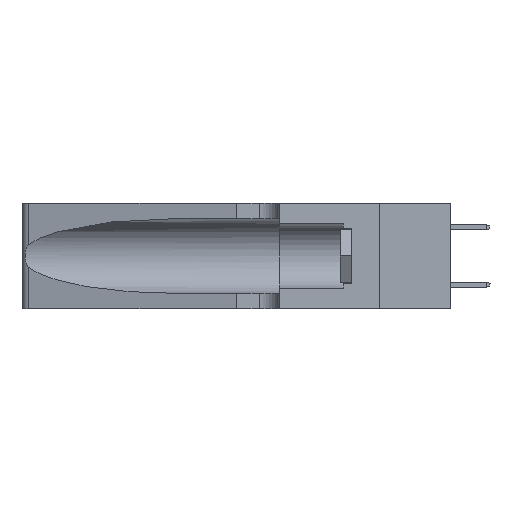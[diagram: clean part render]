
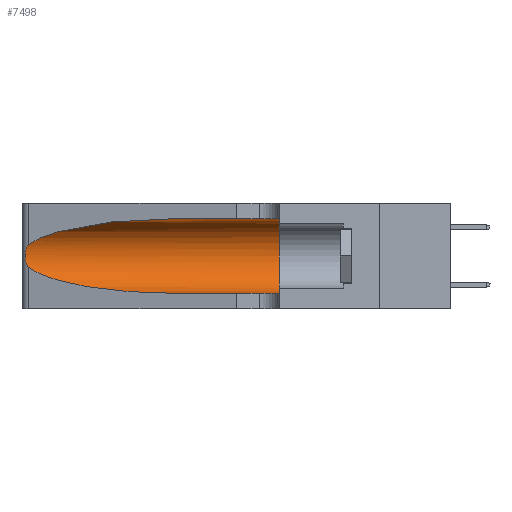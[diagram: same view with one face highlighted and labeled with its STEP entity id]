
A CAD part, left-side view. The second image highlights one B-rep face of the part: STEP entity #7498.
In plain terms, the highlighted cylindrical face has radius 3.308 mm (diameter 6.617 mm), a partial arc.
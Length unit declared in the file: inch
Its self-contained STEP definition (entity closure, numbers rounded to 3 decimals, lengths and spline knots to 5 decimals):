
#547 = VERTEX_POINT ( 'NONE', #1142 ) ;
#1142 = CARTESIAN_POINT ( 'NONE',  ( 0.1305, 0.35, 0.31525 ) ) ;
#2808 = EDGE_LOOP ( 'NONE', ( #38016, #16849, #42690, #29971, #17967, #29332 ) ) ;
#3429 = CARTESIAN_POINT ( 'NONE',  ( 0.25789, 1.23486, 0.15765 ) ) ;
#3972 = CARTESIAN_POINT ( 'NONE',  ( 0.1305, 0.35, 0.05475 ) ) ;
#4000 = FACE_OUTER_BOUND ( 'NONE', #2808, .T. ) ;
#4314 = LINE ( 'NONE', #31258, #21707 ) ;
#4400 = VERTEX_POINT ( 'NONE', #43314 ) ;
#4845 = VERTEX_POINT ( 'NONE', #33265 ) ;
#5397 = CARTESIAN_POINT ( 'NONE',  ( 0.25487, 1.22718, 0.14631 ) ) ;
#5661 = DIRECTION ( 'NONE',  ( 0., 0., 1. ) ) ;
#5883 = CARTESIAN_POINT ( 'NONE',  ( 0.1305, 0.35, 0.185 ) ) ;
#6514 = CARTESIAN_POINT ( 'NONE',  ( 0.25487, 1.22718, 0.22369 ) ) ;
#7188 = CARTESIAN_POINT ( 'NONE',  ( 0.26075, 1.23896, 0.19203 ) ) ;
#7498 = ADVANCED_FACE ( 'NONE', ( #4000 ), #20192, .F. ) ;
#9838 = CARTESIAN_POINT ( 'NONE',  ( 0.18966, 0.96281, 0.31525 ) ) ;
#10511 = CARTESIAN_POINT ( 'NONE',  ( 0.26075, 1.23896, 0.178 ) ) ;
#10900 =( BOUNDED_CURVE ( )  B_SPLINE_CURVE ( 3, ( #19820, #9838, #40145, #18957 ),
 .UNSPECIFIED., .F., .T. ) 
 B_SPLINE_CURVE_WITH_KNOTS ( ( 4, 4 ),
 ( 1.5708, 2.84003 ),
 .UNSPECIFIED. ) 
 CURVE ( )  GEOMETRIC_REPRESENTATION_ITEM ( )  RATIONAL_B_SPLINE_CURVE ( ( 1., 0.87, 0.87, 1. ) ) 
 REPRESENTATION_ITEM ( '' )  );
#13838 = CARTESIAN_POINT ( 'NONE',  ( 0.25639, 1.23184, 0.21858 ) ) ;
#14040 = CARTESIAN_POINT ( 'NONE',  ( 0.26018, 1.23835, 0.19895 ) ) ;
#14261 = CARTESIAN_POINT ( 'NONE',  ( 0.25854, 1.2359, 0.20912 ) ) ;
#16284 = LINE ( 'NONE', #29519, #17554 ) ;
#16849 = ORIENTED_EDGE ( 'NONE', *, *, #32313, .T. ) ;
#16871 = DIRECTION ( 'NONE',  ( 0., 0., -1. ) ) ;
#16875 = CARTESIAN_POINT ( 'NONE',  ( 0.25487, 1.22718, 0.14631 ) ) ;
#17175 = CARTESIAN_POINT ( 'NONE',  ( 0.25555, 1.22994, 0.2215 ) ) ;
#17521 = CARTESIAN_POINT ( 'NONE',  ( 0.1305, 1.61858, 0.185 ) ) ;
#17554 = VECTOR ( 'NONE', #43019, 39.37008 ) ;
#17967 = ORIENTED_EDGE ( 'NONE', *, *, #40953, .F. ) ;
#18218 = VERTEX_POINT ( 'NONE', #16875 ) ;
#18957 = CARTESIAN_POINT ( 'NONE',  ( 0.25487, 1.22718, 0.22369 ) ) ;
#19820 = CARTESIAN_POINT ( 'NONE',  ( 0.1305, 0.72297, 0.31525 ) ) ;
#20192 = CYLINDRICAL_SURFACE ( 'NONE', #36225, 0.13025 ) ;
#21707 = VECTOR ( 'NONE', #34783, 39.37008 ) ;
#23091 =( BOUNDED_CURVE ( )  B_SPLINE_CURVE ( 3, ( #5397, #29693, #42543, #25504 ),
 .UNSPECIFIED., .F., .T. ) 
 B_SPLINE_CURVE_WITH_KNOTS ( ( 4, 4 ),
 ( 3.44316, 4.71239 ),
 .UNSPECIFIED. ) 
 CURVE ( )  GEOMETRIC_REPRESENTATION_ITEM ( )  RATIONAL_B_SPLINE_CURVE ( ( 1., 0.87, 0.87, 1. ) ) 
 REPRESENTATION_ITEM ( '' )  );
#23792 = CARTESIAN_POINT ( 'NONE',  ( 0.25639, 1.23186, 0.15144 ) ) ;
#25504 = CARTESIAN_POINT ( 'NONE',  ( 0.1305, 0.72297, 0.05475 ) ) ;
#25898 = VERTEX_POINT ( 'NONE', #6514 ) ;
#27283 = CARTESIAN_POINT ( 'NONE',  ( 0.25787, 1.23484, 0.2124 ) ) ;
#29332 = ORIENTED_EDGE ( 'NONE', *, *, #34893, .F. ) ;
#29519 = CARTESIAN_POINT ( 'NONE',  ( 0.1305, 1.61858, 0.31525 ) ) ;
#29693 = CARTESIAN_POINT ( 'NONE',  ( 0.2373, 1.15595, 0.08982 ) ) ;
#29971 = ORIENTED_EDGE ( 'NONE', *, *, #33313, .T. ) ;
#30176 = CARTESIAN_POINT ( 'NONE',  ( 0.25555, 1.22993, 0.14849 ) ) ;
#30943 = DIRECTION ( 'NONE',  ( 0., -1., 0. ) ) ;
#31028 = CARTESIAN_POINT ( 'NONE',  ( 0.25487, 1.22718, 0.22369 ) ) ;
#31030 = B_SPLINE_CURVE_WITH_KNOTS ( 'NONE', 3,
 ( #31028, #17175, #13838, #27283, #14261, #14040, #7188, #10511, #37449, #40590, #3429, #23792, #30176, #37234 ),
 .UNSPECIFIED., .F., .F.,
 ( 4, 2, 2, 2, 2, 2, 4 ),
 ( 0., 0.00027, 0.00053, 0.00107, 0.0016, 0.00187, 0.00214 ),
 .UNSPECIFIED. ) ;
#31258 = CARTESIAN_POINT ( 'NONE',  ( 0.1305, 1.61858, 0.05475 ) ) ;
#31313 = EDGE_CURVE ( 'NONE', #18218, #4845, #23091, .T. ) ;
#31614 = CIRCLE ( 'NONE', #37993, 0.13025 ) ;
#32012 = VERTEX_POINT ( 'NONE', #3972 ) ;
#32313 = EDGE_CURVE ( 'NONE', #25898, #18218, #31030, .T. ) ;
#33265 = CARTESIAN_POINT ( 'NONE',  ( 0.1305, 0.72297, 0.05475 ) ) ;
#33313 = EDGE_CURVE ( 'NONE', #4845, #32012, #4314, .T. ) ;
#34783 = DIRECTION ( 'NONE',  ( 0., -1., 0. ) ) ;
#34893 = EDGE_CURVE ( 'NONE', #4400, #547, #16284, .T. ) ;
#36225 = AXIS2_PLACEMENT_3D ( 'NONE', #17521, #30943, #16871 ) ;
#36584 = DIRECTION ( 'NONE',  ( 0., 1., 0. ) ) ;
#37234 = CARTESIAN_POINT ( 'NONE',  ( 0.25487, 1.22718, 0.14631 ) ) ;
#37449 = CARTESIAN_POINT ( 'NONE',  ( 0.26017, 1.23833, 0.17102 ) ) ;
#37993 = AXIS2_PLACEMENT_3D ( 'NONE', #5883, #36584, #5661 ) ;
#38016 = ORIENTED_EDGE ( 'NONE', *, *, #39706, .T. ) ;
#39706 = EDGE_CURVE ( 'NONE', #4400, #25898, #10900, .T. ) ;
#40145 = CARTESIAN_POINT ( 'NONE',  ( 0.2373, 1.15595, 0.28018 ) ) ;
#40590 = CARTESIAN_POINT ( 'NONE',  ( 0.25856, 1.23593, 0.16098 ) ) ;
#40953 = EDGE_CURVE ( 'NONE', #547, #32012, #31614, .T. ) ;
#42543 = CARTESIAN_POINT ( 'NONE',  ( 0.18966, 0.96281, 0.05475 ) ) ;
#42690 = ORIENTED_EDGE ( 'NONE', *, *, #31313, .T. ) ;
#43019 = DIRECTION ( 'NONE',  ( 0., -1., 0. ) ) ;
#43314 = CARTESIAN_POINT ( 'NONE',  ( 0.1305, 0.72297, 0.31525 ) ) ;
